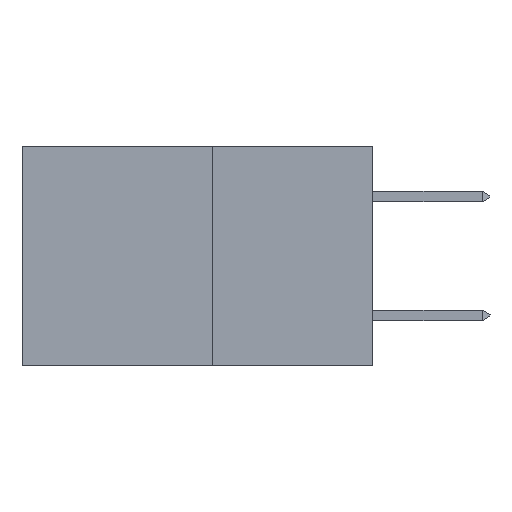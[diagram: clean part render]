
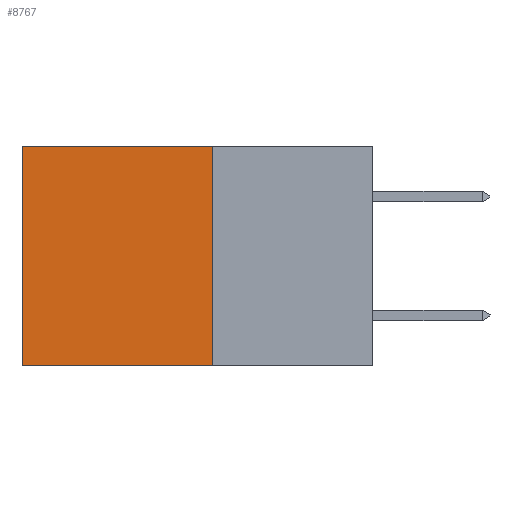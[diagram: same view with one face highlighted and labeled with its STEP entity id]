
A CAD part, left-side view. The second image highlights one B-rep face of the part: STEP entity #8767.
In plain terms, the highlighted planar face has unit normal (-1, 0, 0).
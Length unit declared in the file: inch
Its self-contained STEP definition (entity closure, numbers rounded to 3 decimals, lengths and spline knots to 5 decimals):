
#311 = VECTOR ( 'NONE', #21563, 39.37008 ) ;
#1403 = ORIENTED_EDGE ( 'NONE', *, *, #30976, .T. ) ;
#2530 = LINE ( 'NONE', #10818, #29192 ) ;
#3257 = DIRECTION ( 'NONE',  ( 0., 0., -1. ) ) ;
#4095 = EDGE_CURVE ( 'NONE', #15672, #28553, #25768, .T. ) ;
#4251 = EDGE_CURVE ( 'NONE', #13393, #17882, #7142, .T. ) ;
#5559 = CARTESIAN_POINT ( 'NONE',  ( 0.277, 0.27, 0. ) ) ;
#5618 = LINE ( 'NONE', #31563, #31435 ) ;
#7142 = LINE ( 'NONE', #21643, #311 ) ;
#8767 = ADVANCED_FACE ( 'NONE', ( #26669 ), #13012, .F. ) ;
#9712 = ORIENTED_EDGE ( 'NONE', *, *, #4251, .T. ) ;
#10818 = CARTESIAN_POINT ( 'NONE',  ( 0.277, 0.59, -0.37 ) ) ;
#11382 = DIRECTION ( 'NONE',  ( 0., 0., -1. ) ) ;
#11424 = DIRECTION ( 'NONE',  ( 1., 0., 0. ) ) ;
#11527 = CARTESIAN_POINT ( 'NONE',  ( 0.277, 0.27, -0.37 ) ) ;
#11954 = VECTOR ( 'NONE', #28104, 39.37008 ) ;
#13012 = PLANE ( 'NONE',  #13743 ) ;
#13393 = VERTEX_POINT ( 'NONE', #5559 ) ;
#13743 = AXIS2_PLACEMENT_3D ( 'NONE', #11527, #11424, #11382 ) ;
#15672 = VERTEX_POINT ( 'NONE', #26196 ) ;
#17882 = VERTEX_POINT ( 'NONE', #31124 ) ;
#21323 = ORIENTED_EDGE ( 'NONE', *, *, #28865, .F. ) ;
#21563 = DIRECTION ( 'NONE',  ( 0., 1., 0. ) ) ;
#21643 = CARTESIAN_POINT ( 'NONE',  ( 0.277, 0.27, 0. ) ) ;
#23825 = DIRECTION ( 'NONE',  ( 0., 0., -1. ) ) ;
#25768 = LINE ( 'NONE', #29145, #11954 ) ;
#26147 = EDGE_LOOP ( 'NONE', ( #1403, #31016, #21323, #9712 ) ) ;
#26196 = CARTESIAN_POINT ( 'NONE',  ( 0.277, 0.27, -0.37 ) ) ;
#26669 = FACE_OUTER_BOUND ( 'NONE', #26147, .T. ) ;
#28104 = DIRECTION ( 'NONE',  ( 0., 1., 0. ) ) ;
#28553 = VERTEX_POINT ( 'NONE', #30584 ) ;
#28865 = EDGE_CURVE ( 'NONE', #13393, #15672, #5618, .T. ) ;
#29145 = CARTESIAN_POINT ( 'NONE',  ( 0.277, 0.27, -0.37 ) ) ;
#29192 = VECTOR ( 'NONE', #23825, 39.37008 ) ;
#30584 = CARTESIAN_POINT ( 'NONE',  ( 0.277, 0.59, -0.37 ) ) ;
#30976 = EDGE_CURVE ( 'NONE', #17882, #28553, #2530, .T. ) ;
#31016 = ORIENTED_EDGE ( 'NONE', *, *, #4095, .F. ) ;
#31124 = CARTESIAN_POINT ( 'NONE',  ( 0.277, 0.59, 0. ) ) ;
#31435 = VECTOR ( 'NONE', #3257, 39.37008 ) ;
#31563 = CARTESIAN_POINT ( 'NONE',  ( 0.277, 0.27, -0.37 ) ) ;
